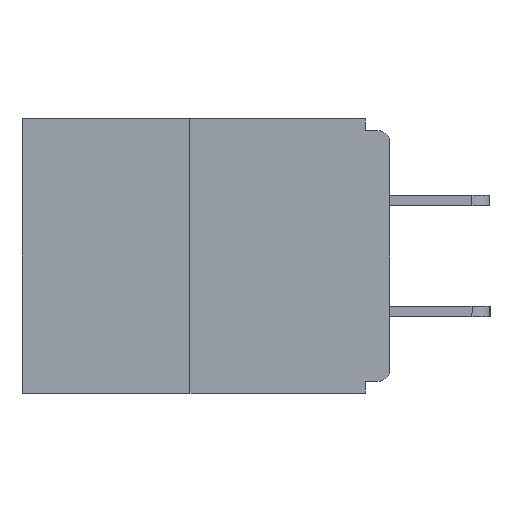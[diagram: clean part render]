
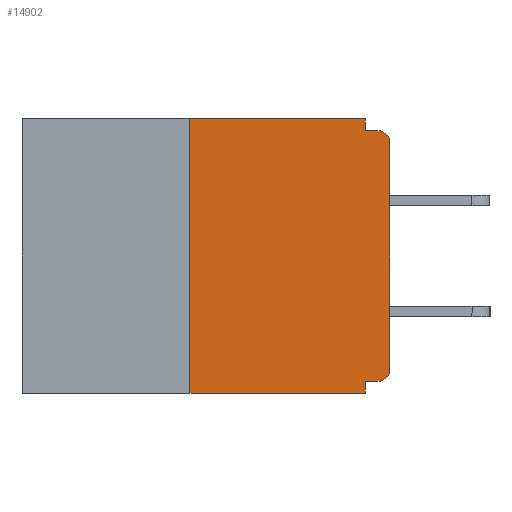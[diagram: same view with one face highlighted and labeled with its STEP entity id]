
A CAD part, left-side view. The second image highlights one B-rep face of the part: STEP entity #14902.
In plain terms, the highlighted planar face has unit normal (-1, 0, 0).
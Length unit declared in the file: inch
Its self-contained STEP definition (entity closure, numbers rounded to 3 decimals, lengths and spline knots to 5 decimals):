
#172 = EDGE_LOOP ( 'NONE', ( #16802, #23244, #24754, #4106, #1766, #9150, #1553, #23003, #11657, #16723 ) ) ;
#333 = VERTEX_POINT ( 'NONE', #20987 ) ;
#1553 = ORIENTED_EDGE ( 'NONE', *, *, #10662, .T. ) ;
#1766 = ORIENTED_EDGE ( 'NONE', *, *, #24455, .F. ) ;
#2037 = VECTOR ( 'NONE', #11767, 39.37008 ) ;
#2144 = VERTEX_POINT ( 'NONE', #14186 ) ;
#2186 = DIRECTION ( 'NONE',  ( 0., -1., 0. ) ) ;
#2705 = DIRECTION ( 'NONE',  ( -1., 0., 0. ) ) ;
#2803 = CARTESIAN_POINT ( 'NONE',  ( 0., 0.031, -0.343 ) ) ;
#3557 = DIRECTION ( 'NONE',  ( 0., 0., -1. ) ) ;
#3563 = AXIS2_PLACEMENT_3D ( 'NONE', #9002, #2705, #23165 ) ;
#3605 = VECTOR ( 'NONE', #4717, 39.37008 ) ;
#4032 = EDGE_CURVE ( 'NONE', #8311, #12280, #22894, .T. ) ;
#4106 = ORIENTED_EDGE ( 'NONE', *, *, #23043, .F. ) ;
#4474 = EDGE_CURVE ( 'NONE', #2144, #26149, #26334, .T. ) ;
#4609 = CARTESIAN_POINT ( 'NONE',  ( 0., 0., -0.328 ) ) ;
#4717 = DIRECTION ( 'NONE',  ( 0., 0., 1. ) ) ;
#5028 = EDGE_CURVE ( 'NONE', #26149, #333, #7676, .T. ) ;
#5286 = EDGE_CURVE ( 'NONE', #6166, #333, #15960, .T. ) ;
#5444 = CARTESIAN_POINT ( 'NONE',  ( 0., 0.25, 0. ) ) ;
#5519 = CARTESIAN_POINT ( 'NONE',  ( 0., 0.015, -0.313 ) ) ;
#5845 = CARTESIAN_POINT ( 'NONE',  ( 0., 0., -0.313 ) ) ;
#6166 = VERTEX_POINT ( 'NONE', #13215 ) ;
#6188 = VERTEX_POINT ( 'NONE', #21391 ) ;
#6330 = EDGE_CURVE ( 'NONE', #6188, #14390, #22578, .T. ) ;
#7256 = CARTESIAN_POINT ( 'NONE',  ( 0., 0.031, -0.328 ) ) ;
#7676 = LINE ( 'NONE', #14292, #18210 ) ;
#8311 = VERTEX_POINT ( 'NONE', #25592 ) ;
#8749 = CARTESIAN_POINT ( 'NONE',  ( 0., 0.25, 0. ) ) ;
#9002 = CARTESIAN_POINT ( 'NONE',  ( 0., 0.015, -0.03 ) ) ;
#9148 = VERTEX_POINT ( 'NONE', #7256 ) ;
#9150 = ORIENTED_EDGE ( 'NONE', *, *, #4032, .T. ) ;
#10466 = CARTESIAN_POINT ( 'NONE',  ( 0., 0.46, 0. ) ) ;
#10574 = FACE_OUTER_BOUND ( 'NONE', #172, .T. ) ;
#10662 = EDGE_CURVE ( 'NONE', #12280, #6166, #15046, .T. ) ;
#11307 = LINE ( 'NONE', #20865, #12572 ) ;
#11318 = LINE ( 'NONE', #8749, #20562 ) ;
#11500 = DIRECTION ( 'NONE',  ( 0., -1., 0. ) ) ;
#11657 = ORIENTED_EDGE ( 'NONE', *, *, #5028, .F. ) ;
#11767 = DIRECTION ( 'NONE',  ( 0., 0., -1. ) ) ;
#12280 = VERTEX_POINT ( 'NONE', #5845 ) ;
#12495 = EDGE_CURVE ( 'NONE', #6188, #25892, #11318, .T. ) ;
#12572 = VECTOR ( 'NONE', #11500, 39.37008 ) ;
#12680 = DIRECTION ( 'NONE',  ( 1., 0., 0. ) ) ;
#12831 = AXIS2_PLACEMENT_3D ( 'NONE', #5519, #19753, #3557 ) ;
#13215 = CARTESIAN_POINT ( 'NONE',  ( 0., 0., -0.03 ) ) ;
#14186 = CARTESIAN_POINT ( 'NONE',  ( 0., 0.031, 0. ) ) ;
#14292 = CARTESIAN_POINT ( 'NONE',  ( 0., 0., -0.015 ) ) ;
#14390 = VERTEX_POINT ( 'NONE', #2803 ) ;
#14664 = CARTESIAN_POINT ( 'NONE',  ( 0., 0., 0. ) ) ;
#14881 = VECTOR ( 'NONE', #26098, 39.37008 ) ;
#14902 = ADVANCED_FACE ( 'NONE', ( #10574 ), #18468, .F. ) ;
#15046 = LINE ( 'NONE', #14664, #3605 ) ;
#15960 = CIRCLE ( 'NONE', #3563, 0.015 ) ;
#16723 = ORIENTED_EDGE ( 'NONE', *, *, #4474, .F. ) ;
#16802 = ORIENTED_EDGE ( 'NONE', *, *, #20693, .F. ) ;
#17819 = CARTESIAN_POINT ( 'NONE',  ( 0., 0.031, -0.343 ) ) ;
#17838 = VECTOR ( 'NONE', #20989, 39.37008 ) ;
#18210 = VECTOR ( 'NONE', #2186, 39.37008 ) ;
#18468 = PLANE ( 'NONE',  #25552 ) ;
#18732 = DIRECTION ( 'NONE',  ( 0., 0., -1. ) ) ;
#19753 = DIRECTION ( 'NONE',  ( -1., 0., 0. ) ) ;
#19855 = CARTESIAN_POINT ( 'NONE',  ( 0., 0.46, -0.343 ) ) ;
#20186 = CARTESIAN_POINT ( 'NONE',  ( 0., 0.031, -0.015 ) ) ;
#20562 = VECTOR ( 'NONE', #23340, 39.37008 ) ;
#20693 = EDGE_CURVE ( 'NONE', #25892, #2144, #11307, .T. ) ;
#20865 = CARTESIAN_POINT ( 'NONE',  ( 0., 0.46, 0. ) ) ;
#20987 = CARTESIAN_POINT ( 'NONE',  ( 0., 0.015, -0.015 ) ) ;
#20989 = DIRECTION ( 'NONE',  ( 0., 1., 0. ) ) ;
#21391 = CARTESIAN_POINT ( 'NONE',  ( 0., 0.25, -0.343 ) ) ;
#21648 = LINE ( 'NONE', #4609, #17838 ) ;
#21796 = LINE ( 'NONE', #17819, #2037 ) ;
#22578 = LINE ( 'NONE', #19855, #25733 ) ;
#22894 = CIRCLE ( 'NONE', #12831, 0.015 ) ;
#23003 = ORIENTED_EDGE ( 'NONE', *, *, #5286, .T. ) ;
#23043 = EDGE_CURVE ( 'NONE', #9148, #14390, #21796, .T. ) ;
#23165 = DIRECTION ( 'NONE',  ( 0., 0., -1. ) ) ;
#23244 = ORIENTED_EDGE ( 'NONE', *, *, #12495, .F. ) ;
#23340 = DIRECTION ( 'NONE',  ( 0., 0., 1. ) ) ;
#23878 = CARTESIAN_POINT ( 'NONE',  ( 0., 0.031, 0. ) ) ;
#24455 = EDGE_CURVE ( 'NONE', #8311, #9148, #21648, .T. ) ;
#24754 = ORIENTED_EDGE ( 'NONE', *, *, #6330, .T. ) ;
#25552 = AXIS2_PLACEMENT_3D ( 'NONE', #10466, #12680, #18732 ) ;
#25592 = CARTESIAN_POINT ( 'NONE',  ( 0., 0.015, -0.328 ) ) ;
#25733 = VECTOR ( 'NONE', #25967, 39.37008 ) ;
#25892 = VERTEX_POINT ( 'NONE', #5444 ) ;
#25967 = DIRECTION ( 'NONE',  ( 0., -1., 0. ) ) ;
#26098 = DIRECTION ( 'NONE',  ( 0., 0., -1. ) ) ;
#26149 = VERTEX_POINT ( 'NONE', #20186 ) ;
#26334 = LINE ( 'NONE', #23878, #14881 ) ;
